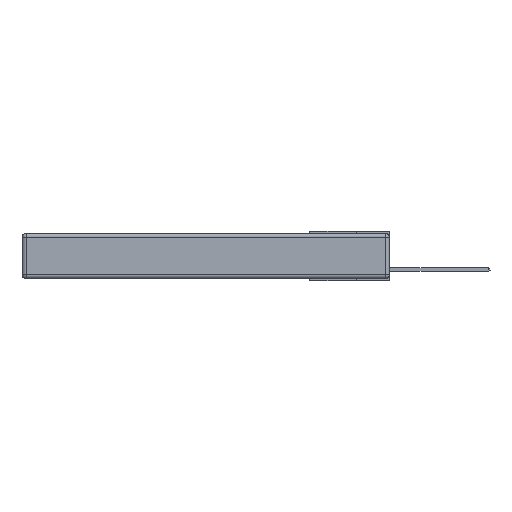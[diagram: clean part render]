
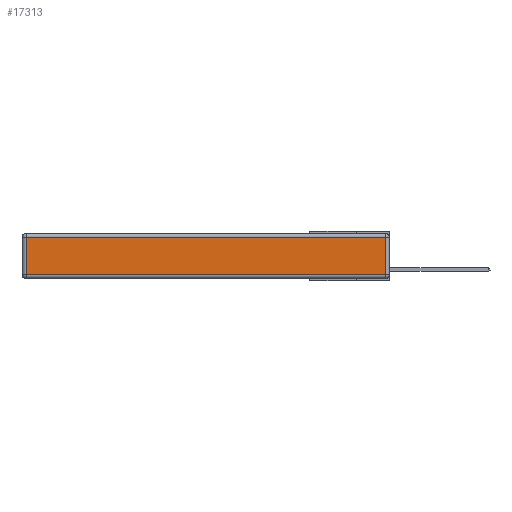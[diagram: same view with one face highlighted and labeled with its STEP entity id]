
A CAD part, left-side view. The second image highlights one B-rep face of the part: STEP entity #17313.
In plain terms, the highlighted planar face has unit normal (-1, 0, 0).
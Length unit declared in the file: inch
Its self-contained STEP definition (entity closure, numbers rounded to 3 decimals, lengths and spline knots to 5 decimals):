
#594 = VERTEX_POINT ( 'NONE', #20612 ) ;
#822 = VECTOR ( 'NONE', #18621, 39.37008 ) ;
#2053 = FACE_OUTER_BOUND ( 'NONE', #6913, .T. ) ;
#2576 = PLANE ( 'NONE',  #18432 ) ;
#3709 = DIRECTION ( 'NONE',  ( 0., 1., 0. ) ) ;
#4369 = ORIENTED_EDGE ( 'NONE', *, *, #17133, .T. ) ;
#4518 = DIRECTION ( 'NONE',  ( 0., 0., 1. ) ) ;
#4939 = LINE ( 'NONE', #21388, #8376 ) ;
#5837 = CARTESIAN_POINT ( 'NONE',  ( 0., 2.72, -0.313 ) ) ;
#6913 = EDGE_LOOP ( 'NONE', ( #25676, #21317, #11134, #4369 ) ) ;
#8376 = VECTOR ( 'NONE', #12663, 39.37008 ) ;
#9720 = CARTESIAN_POINT ( 'NONE',  ( 0., 2.72, -0.343 ) ) ;
#11126 = CARTESIAN_POINT ( 'NONE',  ( 0., 0., -0.343 ) ) ;
#11134 = ORIENTED_EDGE ( 'NONE', *, *, #15781, .T. ) ;
#11659 = LINE ( 'NONE', #20880, #22303 ) ;
#12663 = DIRECTION ( 'NONE',  ( 0., -1., 0. ) ) ;
#13104 = EDGE_CURVE ( 'NONE', #27026, #13541, #22469, .T. ) ;
#13541 = VERTEX_POINT ( 'NONE', #15587 ) ;
#13839 = CARTESIAN_POINT ( 'NONE',  ( 0., 0.03, -0.313 ) ) ;
#14774 = VECTOR ( 'NONE', #25097, 39.37008 ) ;
#15587 = CARTESIAN_POINT ( 'NONE',  ( 0., 0.03, -0.03 ) ) ;
#15781 = EDGE_CURVE ( 'NONE', #13541, #594, #11659, .T. ) ;
#17133 = EDGE_CURVE ( 'NONE', #594, #17650, #20272, .T. ) ;
#17313 = ADVANCED_FACE ( 'NONE', ( #2053 ), #2576, .T. ) ;
#17650 = VERTEX_POINT ( 'NONE', #5837 ) ;
#18432 = AXIS2_PLACEMENT_3D ( 'NONE', #11126, #20160, #4518 ) ;
#18621 = DIRECTION ( 'NONE',  ( 0., 0., 1. ) ) ;
#20160 = DIRECTION ( 'NONE',  ( -1., 0., 0. ) ) ;
#20272 = LINE ( 'NONE', #9720, #14774 ) ;
#20612 = CARTESIAN_POINT ( 'NONE',  ( 0., 2.72, -0.03 ) ) ;
#20880 = CARTESIAN_POINT ( 'NONE',  ( 0., 2.75, -0.03 ) ) ;
#21317 = ORIENTED_EDGE ( 'NONE', *, *, #13104, .T. ) ;
#21388 = CARTESIAN_POINT ( 'NONE',  ( 0., 0., -0.313 ) ) ;
#22303 = VECTOR ( 'NONE', #3709, 39.37008 ) ;
#22469 = LINE ( 'NONE', #25039, #822 ) ;
#25039 = CARTESIAN_POINT ( 'NONE',  ( 0., 0.03, -0.343 ) ) ;
#25097 = DIRECTION ( 'NONE',  ( 0., 0., -1. ) ) ;
#25676 = ORIENTED_EDGE ( 'NONE', *, *, #27833, .T. ) ;
#27026 = VERTEX_POINT ( 'NONE', #13839 ) ;
#27833 = EDGE_CURVE ( 'NONE', #17650, #27026, #4939, .T. ) ;
